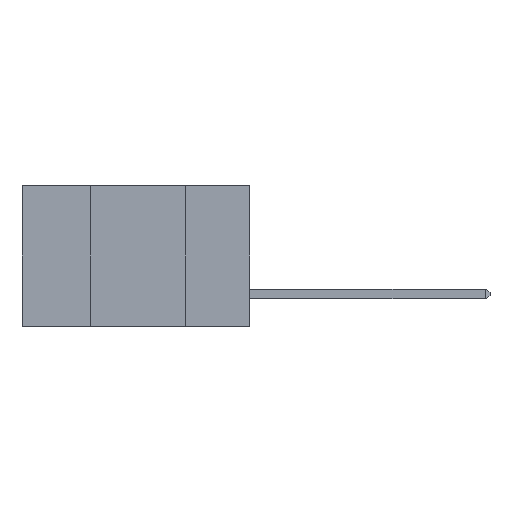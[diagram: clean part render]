
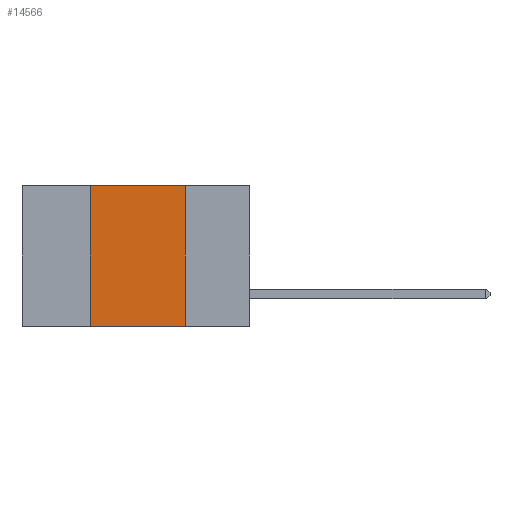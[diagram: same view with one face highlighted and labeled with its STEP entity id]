
A CAD part, left-side view. The second image highlights one B-rep face of the part: STEP entity #14566.
In plain terms, the highlighted planar face has unit normal (-1, 0, 0).
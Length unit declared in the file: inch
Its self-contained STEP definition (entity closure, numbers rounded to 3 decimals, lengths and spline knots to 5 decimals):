
#134 = CARTESIAN_POINT ( 'NONE',  ( 0., 0.42, -0.37 ) ) ;
#1146 = DIRECTION ( 'NONE',  ( 0., 0., 1. ) ) ;
#1579 = CARTESIAN_POINT ( 'NONE',  ( 0., 0.17, 0. ) ) ;
#2847 = VERTEX_POINT ( 'NONE', #5108 ) ;
#2911 = VECTOR ( 'NONE', #7666, 39.37008 ) ;
#3227 = ORIENTED_EDGE ( 'NONE', *, *, #13965, .F. ) ;
#3453 = LINE ( 'NONE', #6070, #2911 ) ;
#3492 = VECTOR ( 'NONE', #15160, 39.37008 ) ;
#3735 = VERTEX_POINT ( 'NONE', #134 ) ;
#5108 = CARTESIAN_POINT ( 'NONE',  ( 0., 0.17, -0.37 ) ) ;
#5381 = CARTESIAN_POINT ( 'NONE',  ( 0., 0.6, -0.37 ) ) ;
#5528 = CARTESIAN_POINT ( 'NONE',  ( 0., 0.42, 0. ) ) ;
#5635 = ORIENTED_EDGE ( 'NONE', *, *, #13189, .F. ) ;
#5882 = ORIENTED_EDGE ( 'NONE', *, *, #18668, .T. ) ;
#6070 = CARTESIAN_POINT ( 'NONE',  ( 0., 0.6, 0. ) ) ;
#7238 = VERTEX_POINT ( 'NONE', #1579 ) ;
#7666 = DIRECTION ( 'NONE',  ( 0., -1., 0. ) ) ;
#7794 = CARTESIAN_POINT ( 'NONE',  ( 0., 0.6, 0. ) ) ;
#7808 = LINE ( 'NONE', #12493, #16455 ) ;
#7857 = DIRECTION ( 'NONE',  ( 1., 0., 0. ) ) ;
#8262 = FACE_OUTER_BOUND ( 'NONE', #11857, .T. ) ;
#11572 = LINE ( 'NONE', #13695, #3492 ) ;
#11857 = EDGE_LOOP ( 'NONE', ( #5635, #3227, #16214, #5882 ) ) ;
#12493 = CARTESIAN_POINT ( 'NONE',  ( 0., 0.42, 0. ) ) ;
#12758 = EDGE_CURVE ( 'NONE', #3735, #19186, #7808, .T. ) ;
#13189 = EDGE_CURVE ( 'NONE', #7238, #2847, #11572, .T. ) ;
#13292 = DIRECTION ( 'NONE',  ( 0., -1., 0. ) ) ;
#13695 = CARTESIAN_POINT ( 'NONE',  ( 0., 0.17, 0. ) ) ;
#13965 = EDGE_CURVE ( 'NONE', #19186, #7238, #3453, .T. ) ;
#14082 = PLANE ( 'NONE',  #14721 ) ;
#14566 = ADVANCED_FACE ( 'NONE', ( #8262 ), #14082, .F. ) ;
#14721 = AXIS2_PLACEMENT_3D ( 'NONE', #7794, #7857, #18422 ) ;
#15160 = DIRECTION ( 'NONE',  ( 0., 0., -1. ) ) ;
#16214 = ORIENTED_EDGE ( 'NONE', *, *, #12758, .F. ) ;
#16455 = VECTOR ( 'NONE', #1146, 39.37008 ) ;
#17434 = VECTOR ( 'NONE', #13292, 39.37008 ) ;
#17878 = LINE ( 'NONE', #5381, #17434 ) ;
#18422 = DIRECTION ( 'NONE',  ( 0., 0., -1. ) ) ;
#18668 = EDGE_CURVE ( 'NONE', #3735, #2847, #17878, .T. ) ;
#19186 = VERTEX_POINT ( 'NONE', #5528 ) ;
